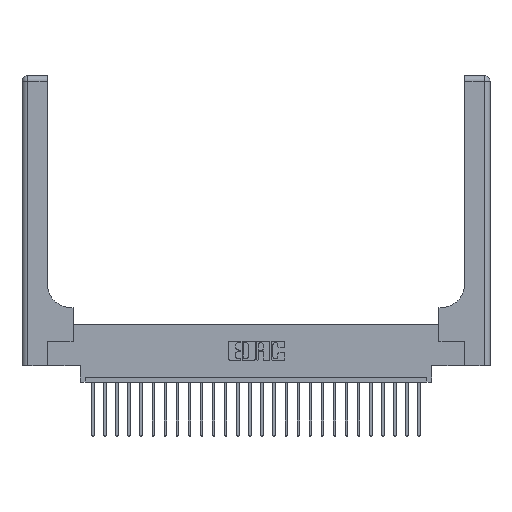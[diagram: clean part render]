
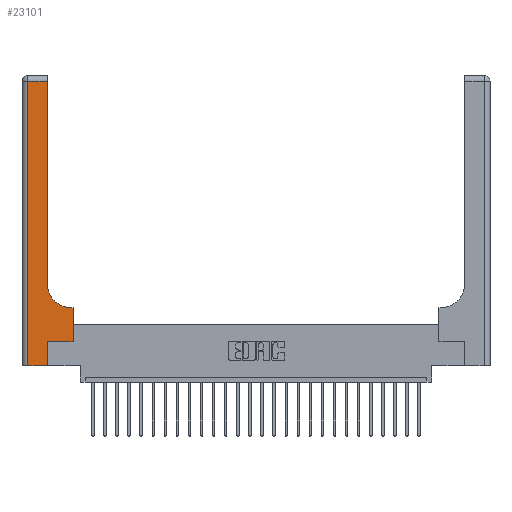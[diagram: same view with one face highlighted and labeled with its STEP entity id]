
A CAD part, top view. The second image highlights one B-rep face of the part: STEP entity #23101.
In plain terms, the highlighted planar face has unit normal (0, 0, 1).
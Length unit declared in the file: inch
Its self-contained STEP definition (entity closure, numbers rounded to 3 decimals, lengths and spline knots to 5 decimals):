
#96 = CARTESIAN_POINT ( 'NONE',  ( 0.265, 0.25, 0.37 ) ) ;
#1429 = VECTOR ( 'NONE', #21123, 39.37008 ) ;
#1535 = CARTESIAN_POINT ( 'NONE',  ( 0.51, 0.6, 0.37 ) ) ;
#1647 = CARTESIAN_POINT ( 'NONE',  ( 0., 3., 0.37 ) ) ;
#1732 = LINE ( 'NONE', #13386, #1429 ) ;
#1753 = VECTOR ( 'NONE', #22167, 39.37008 ) ;
#2817 = CARTESIAN_POINT ( 'NONE',  ( 0.51, 0.85, 0.37 ) ) ;
#3658 = LINE ( 'NONE', #96, #16531 ) ;
#4001 = VECTOR ( 'NONE', #4590, 39.37008 ) ;
#4408 = VECTOR ( 'NONE', #11078, 39.37008 ) ;
#4590 = DIRECTION ( 'NONE',  ( -1., 0., 0. ) ) ;
#4709 = VERTEX_POINT ( 'NONE', #12296 ) ;
#6127 = CARTESIAN_POINT ( 'NONE',  ( 0.06, 0., 0.37 ) ) ;
#6335 = CARTESIAN_POINT ( 'NONE',  ( 0., 0., 0.37 ) ) ;
#6427 = EDGE_CURVE ( 'NONE', #20943, #16271, #23933, .T. ) ;
#6941 = EDGE_LOOP ( 'NONE', ( #9858, #18243, #14994, #9674, #7071, #7056, #14168, #13391, #17522 ) ) ;
#7056 = ORIENTED_EDGE ( 'NONE', *, *, #16300, .T. ) ;
#7071 = ORIENTED_EDGE ( 'NONE', *, *, #21466, .T. ) ;
#7284 = VERTEX_POINT ( 'NONE', #23013 ) ;
#7340 = PLANE ( 'NONE',  #15690 ) ;
#7687 = CARTESIAN_POINT ( 'NONE',  ( 0., 2.94, 0.37 ) ) ;
#7737 = CARTESIAN_POINT ( 'NONE',  ( 0.06, 2.94, 0.37 ) ) ;
#9111 = DIRECTION ( 'NONE',  ( 0., 0., -1. ) ) ;
#9674 = ORIENTED_EDGE ( 'NONE', *, *, #6427, .T. ) ;
#9847 = CARTESIAN_POINT ( 'NONE',  ( 0.265, 0., 0.37 ) ) ;
#9858 = ORIENTED_EDGE ( 'NONE', *, *, #23748, .T. ) ;
#10147 = EDGE_CURVE ( 'NONE', #13678, #20943, #1732, .T. ) ;
#10508 = LINE ( 'NONE', #16206, #11693 ) ;
#11078 = DIRECTION ( 'NONE',  ( 0., 1., 0. ) ) ;
#11341 = CARTESIAN_POINT ( 'NONE',  ( 0.26, 2.94, 0.37 ) ) ;
#11693 = VECTOR ( 'NONE', #22169, 39.37008 ) ;
#12296 = CARTESIAN_POINT ( 'NONE',  ( 0.528, 0.25, 0.37 ) ) ;
#12533 = LINE ( 'NONE', #19902, #15616 ) ;
#12980 = LINE ( 'NONE', #20970, #4408 ) ;
#13190 = AXIS2_PLACEMENT_3D ( 'NONE', #2817, #18503, #21957 ) ;
#13386 = CARTESIAN_POINT ( 'NONE',  ( 0.06, 3., 0.37 ) ) ;
#13391 = ORIENTED_EDGE ( 'NONE', *, *, #14456, .T. ) ;
#13678 = VERTEX_POINT ( 'NONE', #7737 ) ;
#13753 = VERTEX_POINT ( 'NONE', #1535 ) ;
#14168 = ORIENTED_EDGE ( 'NONE', *, *, #14788, .T. ) ;
#14456 = EDGE_CURVE ( 'NONE', #24317, #13753, #14455, .T. ) ;
#14455 = LINE ( 'NONE', #18256, #4001 ) ;
#14788 = EDGE_CURVE ( 'NONE', #4709, #24317, #10508, .T. ) ;
#14994 = ORIENTED_EDGE ( 'NONE', *, *, #10147, .T. ) ;
#15616 = VECTOR ( 'NONE', #21929, 39.37008 ) ;
#15649 = DIRECTION ( 'NONE',  ( -1., 0., 0. ) ) ;
#15690 = AXIS2_PLACEMENT_3D ( 'NONE', #1647, #9111, #24442 ) ;
#16206 = CARTESIAN_POINT ( 'NONE',  ( 0.528, 0.25, 0.37 ) ) ;
#16271 = VERTEX_POINT ( 'NONE', #9847 ) ;
#16300 = EDGE_CURVE ( 'NONE', #7284, #4709, #3658, .T. ) ;
#16531 = VECTOR ( 'NONE', #17362, 39.37008 ) ;
#17362 = DIRECTION ( 'NONE',  ( 1., 0., 0. ) ) ;
#17522 = ORIENTED_EDGE ( 'NONE', *, *, #21099, .T. ) ;
#17640 = CIRCLE ( 'NONE', #13190, 0.25 ) ;
#17677 = LINE ( 'NONE', #7687, #23350 ) ;
#18243 = ORIENTED_EDGE ( 'NONE', *, *, #22384, .T. ) ;
#18256 = CARTESIAN_POINT ( 'NONE',  ( 0.26, 0.6, 0.37 ) ) ;
#18503 = DIRECTION ( 'NONE',  ( 0., 0., -1. ) ) ;
#18864 = FACE_OUTER_BOUND ( 'NONE', #6941, .T. ) ;
#19902 = CARTESIAN_POINT ( 'NONE',  ( 0.265, 0., 0.37 ) ) ;
#20292 = VERTEX_POINT ( 'NONE', #11341 ) ;
#20943 = VERTEX_POINT ( 'NONE', #6127 ) ;
#20970 = CARTESIAN_POINT ( 'NONE',  ( 0.26, 3., 0.37 ) ) ;
#21099 = EDGE_CURVE ( 'NONE', #13753, #22236, #17640, .T. ) ;
#21123 = DIRECTION ( 'NONE',  ( 0., -1., 0. ) ) ;
#21461 = CARTESIAN_POINT ( 'NONE',  ( 0.26, 0.85, 0.37 ) ) ;
#21466 = EDGE_CURVE ( 'NONE', #16271, #7284, #12533, .T. ) ;
#21929 = DIRECTION ( 'NONE',  ( 0., 1., 0. ) ) ;
#21957 = DIRECTION ( 'NONE',  ( 1., 0., 0. ) ) ;
#22167 = DIRECTION ( 'NONE',  ( 1., 0., 0. ) ) ;
#22169 = DIRECTION ( 'NONE',  ( 0., 1., 0. ) ) ;
#22236 = VERTEX_POINT ( 'NONE', #21461 ) ;
#22384 = EDGE_CURVE ( 'NONE', #20292, #13678, #17677, .T. ) ;
#23013 = CARTESIAN_POINT ( 'NONE',  ( 0.265, 0.25, 0.37 ) ) ;
#23101 = ADVANCED_FACE ( 'NONE', ( #18864 ), #7340, .F. ) ;
#23350 = VECTOR ( 'NONE', #15649, 39.37008 ) ;
#23748 = EDGE_CURVE ( 'NONE', #22236, #20292, #12980, .T. ) ;
#23807 = CARTESIAN_POINT ( 'NONE',  ( 0.528, 0.6, 0.37 ) ) ;
#23933 = LINE ( 'NONE', #6335, #1753 ) ;
#24317 = VERTEX_POINT ( 'NONE', #23807 ) ;
#24442 = DIRECTION ( 'NONE',  ( -1., 0., 0. ) ) ;
